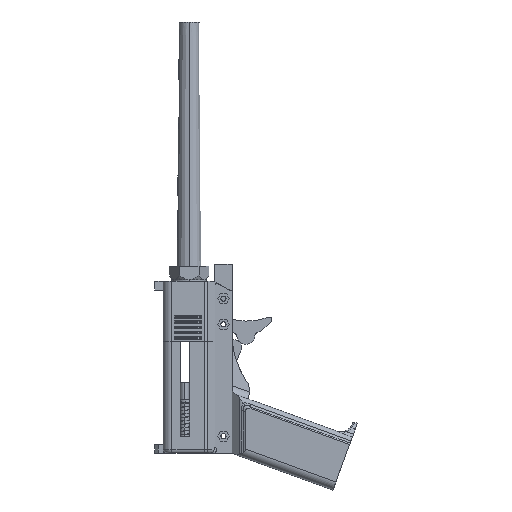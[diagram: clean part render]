
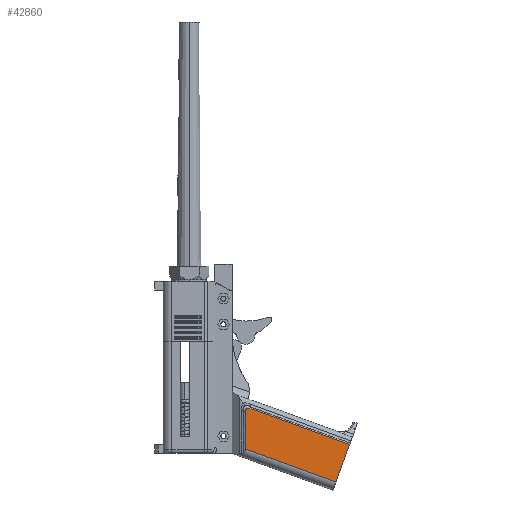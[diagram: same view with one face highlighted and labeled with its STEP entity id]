
A CAD part, left-side view. The second image highlights one B-rep face of the part: STEP entity #42860.
In plain terms, the highlighted face is planar.
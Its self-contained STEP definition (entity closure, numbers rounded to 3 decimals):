
#565 = VECTOR ( 'NONE', #45265, 1000. ) ;
#827 = PLANE ( 'NONE',  #31051 ) ;
#1094 = CARTESIAN_POINT ( 'NONE',  ( 21., 15.474, 42.515 ) ) ;
#5388 = DIRECTION ( 'NONE',  ( -1., 0., 0. ) ) ;
#8070 = EDGE_CURVE ( 'NONE', #44581, #34720, #23215, .T. ) ;
#8893 = VERTEX_POINT ( 'NONE', #40919 ) ;
#11503 = VECTOR ( 'NONE', #46376, 1000. ) ;
#11935 = VERTEX_POINT ( 'NONE', #49317 ) ;
#14968 = ORIENTED_EDGE ( 'NONE', *, *, #18190, .T. ) ;
#18190 = EDGE_CURVE ( 'NONE', #8893, #44581, #29155, .T. ) ;
#18510 = CARTESIAN_POINT ( 'NONE',  ( 21., -11.976, 29.127 ) ) ;
#18678 = DIRECTION ( 'NONE',  ( 0., 0.94, -0.342 ) ) ;
#20160 = CARTESIAN_POINT ( 'NONE',  ( 21., -73.182, 48.297 ) ) ;
#20972 = ORIENTED_EDGE ( 'NONE', *, *, #28373, .T. ) ;
#22351 = CARTESIAN_POINT ( 'NONE',  ( 21., -11.976, 31.433 ) ) ;
#23041 = CARTESIAN_POINT ( 'NONE',  ( 21., -15.331, 29.084 ) ) ;
#23215 =( BOUNDED_CURVE ( )  B_SPLINE_CURVE ( 3, ( #23041, #50145, #18510, #27616 ),
 .UNSPECIFIED., .F., .F. ) 
 B_SPLINE_CURVE_WITH_KNOTS ( ( 4, 4 ),
 ( 5.861, 6.705 ),
 .UNSPECIFIED. ) 
 CURVE ( )  GEOMETRIC_REPRESENTATION_ITEM ( )  RATIONAL_B_SPLINE_CURVE ( ( 1., 0.942, 0.942, 1. ) ) 
 REPRESENTATION_ITEM ( '' )  );
#24953 = LINE ( 'NONE', #1094, #11503 ) ;
#26877 = ORIENTED_EDGE ( 'NONE', *, *, #53854, .T. ) ;
#27616 = CARTESIAN_POINT ( 'NONE',  ( 21., -11.976, 31.433 ) ) ;
#28373 = EDGE_CURVE ( 'NONE', #11935, #53474, #24953, .T. ) ;
#28589 = CARTESIAN_POINT ( 'NONE',  ( 21., -64.669, 71.685 ) ) ;
#29155 = LINE ( 'NONE', #45766, #39726 ) ;
#30908 = ORIENTED_EDGE ( 'NONE', *, *, #8070, .T. ) ;
#31051 = AXIS2_PLACEMENT_3D ( 'NONE', #45918, #5388, #37021 ) ;
#31655 = CARTESIAN_POINT ( 'NONE',  ( 21., -11.976, 0. ) ) ;
#32742 = FACE_OUTER_BOUND ( 'NONE', #57259, .T. ) ;
#34720 = VERTEX_POINT ( 'NONE', #22351 ) ;
#35809 = VECTOR ( 'NONE', #51820, 1000. ) ;
#36654 = LINE ( 'NONE', #31655, #565 ) ;
#37021 = DIRECTION ( 'NONE',  ( 0., 0., 1. ) ) ;
#39726 = VECTOR ( 'NONE', #18678, 1000. ) ;
#40919 = CARTESIAN_POINT ( 'NONE',  ( 21., -72.589, 49.925 ) ) ;
#42860 = ADVANCED_FACE ( 'NONE', ( #32742 ), #827, .F. ) ;
#44581 = VERTEX_POINT ( 'NONE', #57407 ) ;
#45265 = DIRECTION ( 'NONE',  ( 0., 0., 1. ) ) ;
#45766 = CARTESIAN_POINT ( 'NONE',  ( 21., 7.554, 20.755 ) ) ;
#45918 = CARTESIAN_POINT ( 'NONE',  ( 21., 0., 0. ) ) ;
#46376 = DIRECTION ( 'NONE',  ( 0., -0.94, 0.342 ) ) ;
#46396 = LINE ( 'NONE', #20160, #35809 ) ;
#47562 = EDGE_CURVE ( 'NONE', #34720, #11935, #36654, .T. ) ;
#49317 = CARTESIAN_POINT ( 'NONE',  ( 21., -11.976, 52.506 ) ) ;
#50145 = CARTESIAN_POINT ( 'NONE',  ( 21., -13.163, 28.295 ) ) ;
#51820 = DIRECTION ( 'NONE',  ( 0., -0.342, -0.94 ) ) ;
#53474 = VERTEX_POINT ( 'NONE', #28589 ) ;
#53844 = ORIENTED_EDGE ( 'NONE', *, *, #47562, .T. ) ;
#53854 = EDGE_CURVE ( 'NONE', #53474, #8893, #46396, .T. ) ;
#57259 = EDGE_LOOP ( 'NONE', ( #53844, #20972, #26877, #14968, #30908 ) ) ;
#57407 = CARTESIAN_POINT ( 'NONE',  ( 21., -15.331, 29.084 ) ) ;
